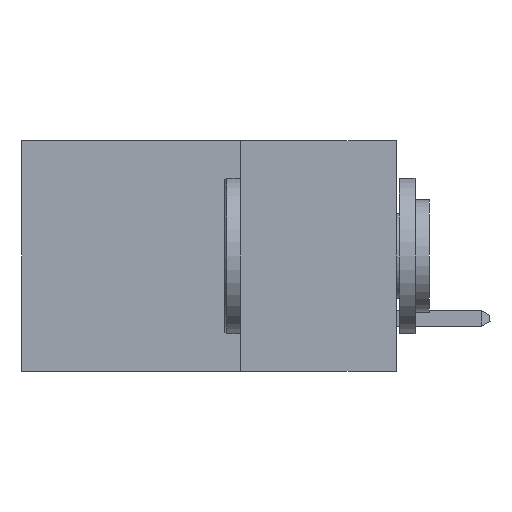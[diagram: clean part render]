
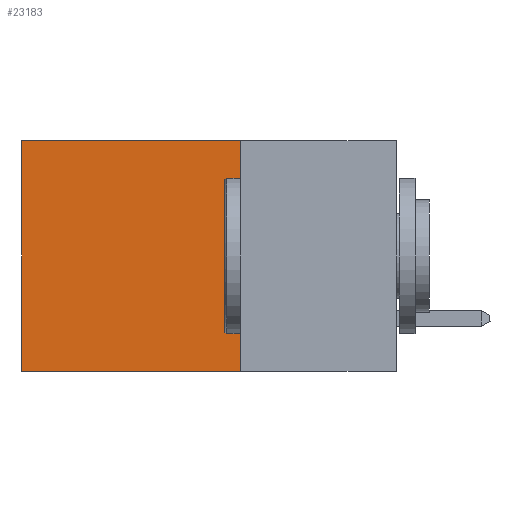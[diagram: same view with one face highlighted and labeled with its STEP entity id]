
A CAD part, left-side view. The second image highlights one B-rep face of the part: STEP entity #23183.
In plain terms, the highlighted planar face has unit normal (-1, 0, 0).
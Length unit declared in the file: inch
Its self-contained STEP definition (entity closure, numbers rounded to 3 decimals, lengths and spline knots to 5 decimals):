
#1903 = VECTOR ( 'NONE', #5717, 39.37008 ) ;
#1972 = EDGE_CURVE ( 'NONE', #8575, #18903, #7239, .T. ) ;
#3272 = ORIENTED_EDGE ( 'NONE', *, *, #20789, .F. ) ;
#4011 = LINE ( 'NONE', #17823, #15388 ) ;
#4674 = VERTEX_POINT ( 'NONE', #16065 ) ;
#5184 = EDGE_CURVE ( 'NONE', #4674, #20158, #4011, .T. ) ;
#5573 = ORIENTED_EDGE ( 'NONE', *, *, #1972, .T. ) ;
#5627 = CARTESIAN_POINT ( 'NONE',  ( 0.298, 0.6, -0.37 ) ) ;
#5717 = DIRECTION ( 'NONE',  ( 0., 0., -1. ) ) ;
#7239 = LINE ( 'NONE', #9984, #17972 ) ;
#7987 = CARTESIAN_POINT ( 'NONE',  ( 0.298, 0.6, 0. ) ) ;
#8575 = VERTEX_POINT ( 'NONE', #22599 ) ;
#9286 = DIRECTION ( 'NONE',  ( 0., 1., 0. ) ) ;
#9984 = CARTESIAN_POINT ( 'NONE',  ( 0.298, 0.25, 0. ) ) ;
#10932 = EDGE_LOOP ( 'NONE', ( #18944, #12445, #3272, #5573 ) ) ;
#12421 = EDGE_CURVE ( 'NONE', #18903, #20158, #26065, .T. ) ;
#12445 = ORIENTED_EDGE ( 'NONE', *, *, #5184, .F. ) ;
#12557 = DIRECTION ( 'NONE',  ( 1., 0., 0. ) ) ;
#12973 = VECTOR ( 'NONE', #26856, 39.37008 ) ;
#15388 = VECTOR ( 'NONE', #17894, 39.37008 ) ;
#16065 = CARTESIAN_POINT ( 'NONE',  ( 0.298, 0.25, -0.37 ) ) ;
#17823 = CARTESIAN_POINT ( 'NONE',  ( 0.298, 0.25, -0.37 ) ) ;
#17894 = DIRECTION ( 'NONE',  ( 0., 1., 0. ) ) ;
#17972 = VECTOR ( 'NONE', #9286, 39.37008 ) ;
#18097 = AXIS2_PLACEMENT_3D ( 'NONE', #26136, #12557, #28413 ) ;
#18903 = VERTEX_POINT ( 'NONE', #24010 ) ;
#18944 = ORIENTED_EDGE ( 'NONE', *, *, #12421, .T. ) ;
#20076 = CARTESIAN_POINT ( 'NONE',  ( 0.298, 0.25, 0. ) ) ;
#20158 = VERTEX_POINT ( 'NONE', #5627 ) ;
#20789 = EDGE_CURVE ( 'NONE', #8575, #4674, #24348, .T. ) ;
#21288 = FACE_OUTER_BOUND ( 'NONE', #10932, .T. ) ;
#21610 = PLANE ( 'NONE',  #18097 ) ;
#22599 = CARTESIAN_POINT ( 'NONE',  ( 0.298, 0.25, 0. ) ) ;
#23183 = ADVANCED_FACE ( 'NONE', ( #21288 ), #21610, .F. ) ;
#24010 = CARTESIAN_POINT ( 'NONE',  ( 0.298, 0.6, 0. ) ) ;
#24348 = LINE ( 'NONE', #20076, #12973 ) ;
#26065 = LINE ( 'NONE', #7987, #1903 ) ;
#26136 = CARTESIAN_POINT ( 'NONE',  ( 0.298, 0.25, 0. ) ) ;
#26856 = DIRECTION ( 'NONE',  ( 0., 0., -1. ) ) ;
#28413 = DIRECTION ( 'NONE',  ( 0., 0., -1. ) ) ;
